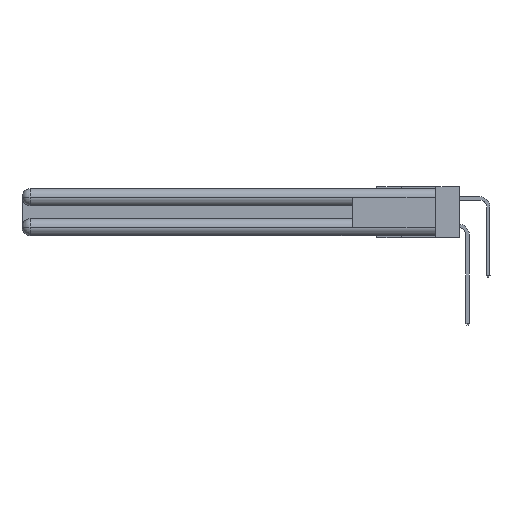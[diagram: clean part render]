
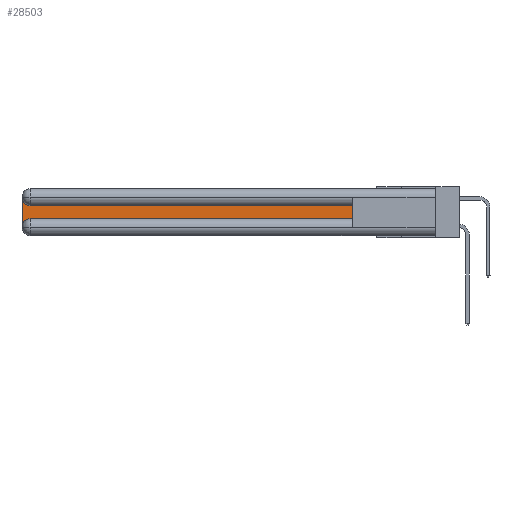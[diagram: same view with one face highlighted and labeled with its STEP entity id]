
A CAD part, left-side view. The second image highlights one B-rep face of the part: STEP entity #28503.
In plain terms, the highlighted planar face has unit normal (-1, 0, 0).
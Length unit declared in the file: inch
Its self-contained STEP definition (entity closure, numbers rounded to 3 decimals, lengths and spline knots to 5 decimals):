
#665 = ORIENTED_EDGE ( 'NONE', *, *, #2642, .T. ) ;
#916 = CARTESIAN_POINT ( 'NONE',  ( 0.075, 2.94, -0.2775 ) ) ;
#1548 = VERTEX_POINT ( 'NONE', #6589 ) ;
#2079 = AXIS2_PLACEMENT_3D ( 'NONE', #27944, #19817, #25413 ) ;
#2642 = EDGE_CURVE ( 'NONE', #35467, #36716, #32036, .T. ) ;
#3074 = CARTESIAN_POINT ( 'NONE',  ( 0.075, 0.6, -0.1225 ) ) ;
#3314 = DIRECTION ( 'NONE',  ( 1., 0., 0. ) ) ;
#3408 = ORIENTED_EDGE ( 'NONE', *, *, #24067, .T. ) ;
#3819 = EDGE_CURVE ( 'NONE', #22045, #7975, #10161, .T. ) ;
#5132 = CIRCLE ( 'NONE', #37054, 0.06 ) ;
#5511 = CARTESIAN_POINT ( 'NONE',  ( 0.075, 0.6, -0.2175 ) ) ;
#5650 = CARTESIAN_POINT ( 'NONE',  ( 0.075, 0.6, -0.2175 ) ) ;
#6067 = CARTESIAN_POINT ( 'NONE',  ( 0.075, 2.94, -0.1225 ) ) ;
#6271 = FACE_OUTER_BOUND ( 'NONE', #28793, .T. ) ;
#6569 = VECTOR ( 'NONE', #8510, 39.37008 ) ;
#6589 = CARTESIAN_POINT ( 'NONE',  ( 0.075, 3., -0.2775 ) ) ;
#7975 = VERTEX_POINT ( 'NONE', #35739 ) ;
#8510 = DIRECTION ( 'NONE',  ( 0., -1., 0. ) ) ;
#10161 = LINE ( 'NONE', #24219, #16497 ) ;
#10603 = ORIENTED_EDGE ( 'NONE', *, *, #15577, .T. ) ;
#11011 = ORIENTED_EDGE ( 'NONE', *, *, #3819, .T. ) ;
#13791 = DIRECTION ( 'NONE',  ( 0., 0., -1. ) ) ;
#13826 = DIRECTION ( 'NONE',  ( 0., 0., -1. ) ) ;
#15577 = EDGE_CURVE ( 'NONE', #7975, #35467, #16859, .T. ) ;
#16377 = CARTESIAN_POINT ( 'NONE',  ( 0.075, 2.94, -0.0625 ) ) ;
#16497 = VECTOR ( 'NONE', #27119, 39.37008 ) ;
#16859 = LINE ( 'NONE', #3074, #20886 ) ;
#19817 = DIRECTION ( 'NONE',  ( 1., 0., 0. ) ) ;
#20306 = DIRECTION ( 'NONE',  ( 0., 1., 0. ) ) ;
#20479 = EDGE_CURVE ( 'NONE', #1548, #35921, #5132, .T. ) ;
#20614 = LINE ( 'NONE', #33237, #30423 ) ;
#20886 = VECTOR ( 'NONE', #20306, 39.37008 ) ;
#22045 = VERTEX_POINT ( 'NONE', #5511 ) ;
#23210 = AXIS2_PLACEMENT_3D ( 'NONE', #16377, #31000, #13826 ) ;
#23636 = DIRECTION ( 'NONE',  ( 0., 0., -1. ) ) ;
#24067 = EDGE_CURVE ( 'NONE', #35921, #22045, #30337, .T. ) ;
#24219 = CARTESIAN_POINT ( 'NONE',  ( 0.075, 0.6, -0.2175 ) ) ;
#25413 = DIRECTION ( 'NONE',  ( 0., 0., -1. ) ) ;
#27119 = DIRECTION ( 'NONE',  ( 0., 0., 1. ) ) ;
#27944 = CARTESIAN_POINT ( 'NONE',  ( 0.075, 3., -0.1225 ) ) ;
#27964 = CARTESIAN_POINT ( 'NONE',  ( 0.075, 2.94, -0.2175 ) ) ;
#28503 = ADVANCED_FACE ( 'NONE', ( #6271 ), #30828, .F. ) ;
#28793 = EDGE_LOOP ( 'NONE', ( #10603, #665, #36232, #35421, #3408, #11011 ) ) ;
#30337 = LINE ( 'NONE', #5650, #6569 ) ;
#30423 = VECTOR ( 'NONE', #13791, 39.37008 ) ;
#30828 = PLANE ( 'NONE',  #2079 ) ;
#31000 = DIRECTION ( 'NONE',  ( 1., 0., 0. ) ) ;
#32036 = CIRCLE ( 'NONE', #23210, 0.06 ) ;
#32442 = CARTESIAN_POINT ( 'NONE',  ( 0.075, 3., -0.0625 ) ) ;
#33237 = CARTESIAN_POINT ( 'NONE',  ( 0.075, 3., -0.2175 ) ) ;
#35421 = ORIENTED_EDGE ( 'NONE', *, *, #20479, .T. ) ;
#35467 = VERTEX_POINT ( 'NONE', #6067 ) ;
#35739 = CARTESIAN_POINT ( 'NONE',  ( 0.075, 0.6, -0.1225 ) ) ;
#35805 = EDGE_CURVE ( 'NONE', #36716, #1548, #20614, .T. ) ;
#35921 = VERTEX_POINT ( 'NONE', #27964 ) ;
#36232 = ORIENTED_EDGE ( 'NONE', *, *, #35805, .T. ) ;
#36716 = VERTEX_POINT ( 'NONE', #32442 ) ;
#37054 = AXIS2_PLACEMENT_3D ( 'NONE', #916, #3314, #23636 ) ;
